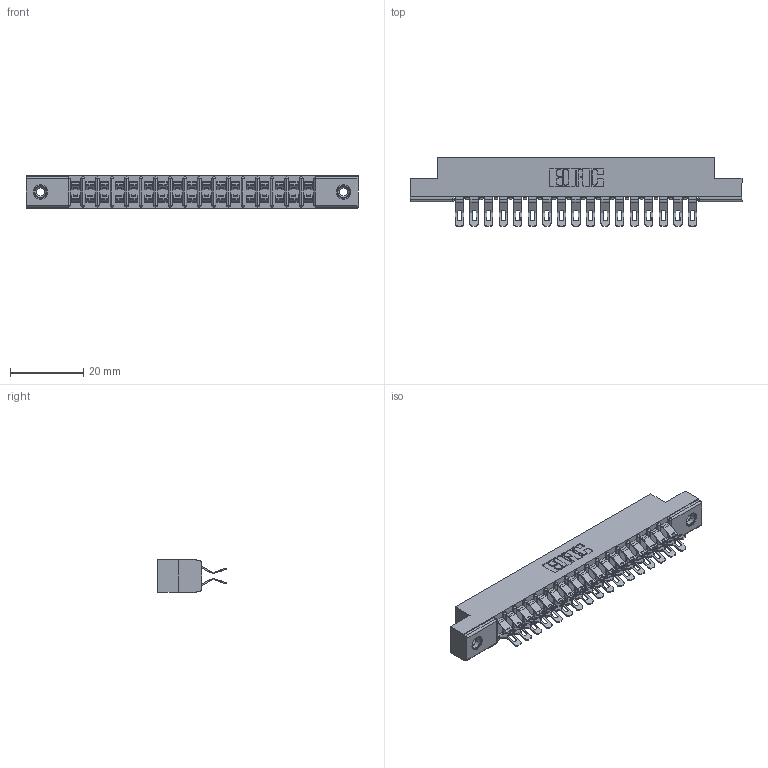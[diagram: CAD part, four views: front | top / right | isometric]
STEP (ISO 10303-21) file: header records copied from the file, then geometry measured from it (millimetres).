
FILE_DESCRIPTION (( 'STEP AP203' ), '1' );
FILE_NAME ('307-034-455-208.STEP', '2020-09-29T16:09:01', ( '' ), ( '' ), 'SwSTEP 2.0', 'SolidWorks 2020', '' );
FILE_SCHEMA (( 'CONFIG_CONTROL_DESIGN' ));
Length unit declared in the file: inch
Products named in the file (4): 345-250-001_345-250-003-102; 307 Part_.156 Dia Mounting Holes; 307-290-001_555; 307-034-455-208
Assembly tree (37 placements, depth 2):
  307-034-455-208
    307 Part_.156 Dia Mounting Holes
    307-290-001_555  x34
    345-250-001_345-250-003-102  x2
Bounding box: 90.37 x 18.75 x 8.71 mm (x, y, z)
Volume: 6006.7 mm3; surface area: 10929.7 mm2
Topology: 37 solids, 37 shells, 2270 faces, 6613 edges, 4306 vertices
Faces by surface type: plane 1258, cylinder 960, sphere 36, cone 12, torus 4
Entity records: 19922 total; most frequent: CARTESIAN_POINT 3256, ORIENTED_EDGE 3220, DIRECTION 3216, EDGE_CURVE 1610, LINE 1212, VECTOR 1212, VERTEX_POINT 1042, AXIS2_PLACEMENT_3D 1002
